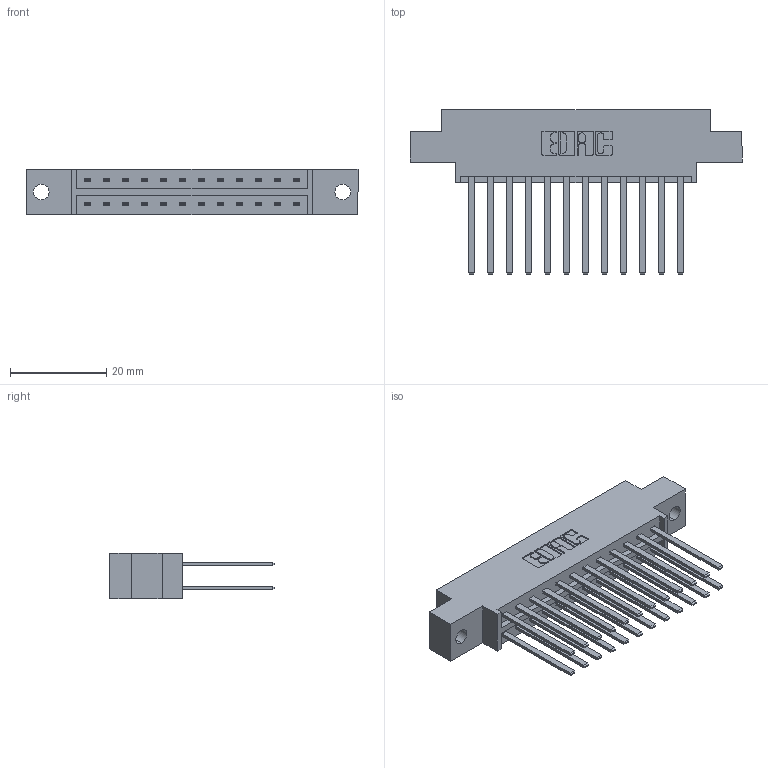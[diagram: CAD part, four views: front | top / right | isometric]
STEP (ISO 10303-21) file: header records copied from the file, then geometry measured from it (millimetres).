
FILE_DESCRIPTION (( 'STEP AP203' ), '1' );
FILE_NAME ('333-024-544-802.STEP', '2018-08-02T11:32:11', ( '' ), ( '' ), 'SwSTEP 2.0', 'SolidWorks 2016', '' );
FILE_SCHEMA (( 'CONFIG_CONTROL_DESIGN' ));
Length unit declared in the file: inch
Products named in the file (3): 333 Part_Offset - .128 Dia; 345-292-001_345-293-144; 333-024-544-802
Assembly tree (25 placements, depth 2):
  333-024-544-802
    333 Part_Offset - .128 Dia
    345-292-001_345-293-144  x24
Bounding box: 69.09 x 34.3 x 9.4 mm (x, y, z)
Volume: 6844.9 mm3; surface area: 8800.7 mm2
Topology: 25 solids, 25 shells, 1222 faces, 3611 edges, 2374 vertices
Faces by surface type: plane 842, cylinder 380
Entity records: 11551 total; most frequent: CARTESIAN_POINT 1950, ORIENTED_EDGE 1886, DIRECTION 1715, EDGE_CURVE 943, LINE 819, VECTOR 819, VERTEX_POINT 626, AXIS2_PLACEMENT_3D 448
